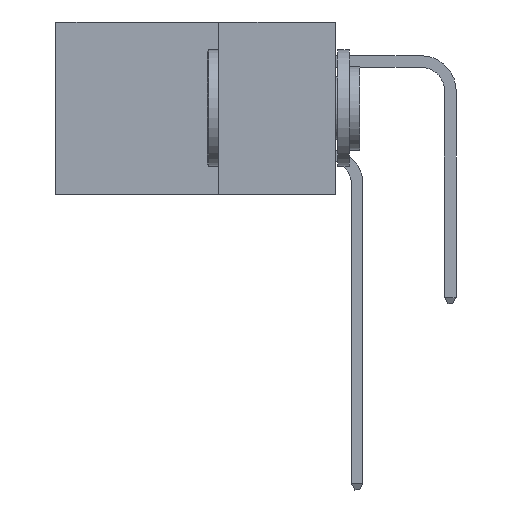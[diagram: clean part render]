
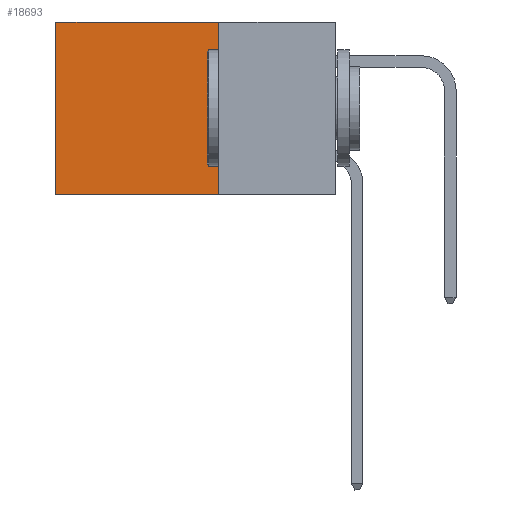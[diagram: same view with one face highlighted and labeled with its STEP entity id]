
A CAD part, left-side view. The second image highlights one B-rep face of the part: STEP entity #18693.
In plain terms, the highlighted planar face has unit normal (-1, 0, 0).
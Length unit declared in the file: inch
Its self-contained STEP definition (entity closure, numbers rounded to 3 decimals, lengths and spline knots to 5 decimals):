
#447 = VERTEX_POINT ( 'NONE', #18054 ) ;
#1331 = DIRECTION ( 'NONE',  ( 0., 1., 0. ) ) ;
#2348 = AXIS2_PLACEMENT_3D ( 'NONE', #6404, #9337, #7768 ) ;
#2359 = ORIENTED_EDGE ( 'NONE', *, *, #17773, .F. ) ;
#2635 = VECTOR ( 'NONE', #1331, 39.37008 ) ;
#3424 = EDGE_CURVE ( 'NONE', #9474, #18336, #3626, .T. ) ;
#3626 = LINE ( 'NONE', #10433, #16904 ) ;
#4248 = LINE ( 'NONE', #11199, #15475 ) ;
#5144 = VECTOR ( 'NONE', #15971, 39.37008 ) ;
#5392 = CARTESIAN_POINT ( 'NONE',  ( 0.2875, 0.25, 0. ) ) ;
#6404 = CARTESIAN_POINT ( 'NONE',  ( 0.2875, 0.25, 0. ) ) ;
#6943 = VERTEX_POINT ( 'NONE', #19037 ) ;
#7066 = CARTESIAN_POINT ( 'NONE',  ( 0.2875, 0.25, -0.37 ) ) ;
#7768 = DIRECTION ( 'NONE',  ( 0., 0., -1. ) ) ;
#8958 = DIRECTION ( 'NONE',  ( 0., 0., -1. ) ) ;
#9066 = EDGE_CURVE ( 'NONE', #9474, #447, #12503, .T. ) ;
#9337 = DIRECTION ( 'NONE',  ( 1., 0., 0. ) ) ;
#9474 = VERTEX_POINT ( 'NONE', #9494 ) ;
#9494 = CARTESIAN_POINT ( 'NONE',  ( 0.2875, 0.25, 0. ) ) ;
#10433 = CARTESIAN_POINT ( 'NONE',  ( 0.2875, 0.25, 0. ) ) ;
#10733 = ORIENTED_EDGE ( 'NONE', *, *, #3424, .F. ) ;
#11199 = CARTESIAN_POINT ( 'NONE',  ( 0.2875, 0.25, -0.37 ) ) ;
#11204 = ORIENTED_EDGE ( 'NONE', *, *, #9066, .T. ) ;
#12503 = LINE ( 'NONE', #5392, #2635 ) ;
#12947 = LINE ( 'NONE', #15839, #5144 ) ;
#13006 = ORIENTED_EDGE ( 'NONE', *, *, #17333, .T. ) ;
#14278 = FACE_OUTER_BOUND ( 'NONE', #15818, .T. ) ;
#14341 = DIRECTION ( 'NONE',  ( 0., 1., 0. ) ) ;
#15335 = PLANE ( 'NONE',  #2348 ) ;
#15475 = VECTOR ( 'NONE', #14341, 39.37008 ) ;
#15818 = EDGE_LOOP ( 'NONE', ( #13006, #2359, #10733, #11204 ) ) ;
#15839 = CARTESIAN_POINT ( 'NONE',  ( 0.2875, 0.6, 0. ) ) ;
#15971 = DIRECTION ( 'NONE',  ( 0., 0., -1. ) ) ;
#16904 = VECTOR ( 'NONE', #8958, 39.37008 ) ;
#17333 = EDGE_CURVE ( 'NONE', #447, #6943, #12947, .T. ) ;
#17773 = EDGE_CURVE ( 'NONE', #18336, #6943, #4248, .T. ) ;
#18054 = CARTESIAN_POINT ( 'NONE',  ( 0.2875, 0.6, 0. ) ) ;
#18336 = VERTEX_POINT ( 'NONE', #7066 ) ;
#18693 = ADVANCED_FACE ( 'NONE', ( #14278 ), #15335, .F. ) ;
#19037 = CARTESIAN_POINT ( 'NONE',  ( 0.2875, 0.6, -0.37 ) ) ;
